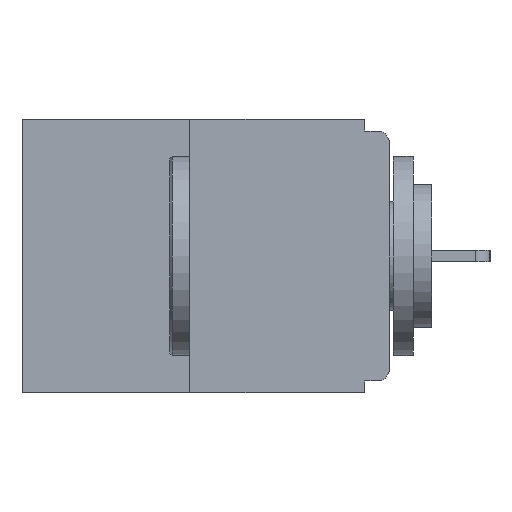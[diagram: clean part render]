
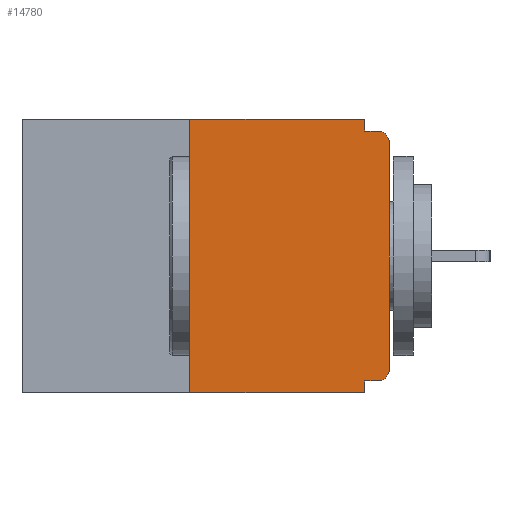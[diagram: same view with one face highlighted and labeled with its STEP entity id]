
A CAD part, left-side view. The second image highlights one B-rep face of the part: STEP entity #14780.
In plain terms, the highlighted planar face has unit normal (-1, 0, 0).
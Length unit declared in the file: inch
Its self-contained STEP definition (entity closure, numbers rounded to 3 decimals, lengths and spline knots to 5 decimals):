
#3 = EDGE_CURVE ( 'NONE', #1493, #1926, #19079, .T. ) ;
#539 = LINE ( 'NONE', #24340, #20192 ) ;
#793 = VECTOR ( 'NONE', #6854, 39.37008 ) ;
#969 = DIRECTION ( 'NONE',  ( 0., 0., 1. ) ) ;
#1248 = DIRECTION ( 'NONE',  ( 0., -1., 0. ) ) ;
#1493 = VERTEX_POINT ( 'NONE', #18992 ) ;
#1844 = EDGE_LOOP ( 'NONE', ( #14877, #3896, #26141, #13266, #27011, #18038, #16383, #17602, #20513, #16211 ) ) ;
#1926 = VERTEX_POINT ( 'NONE', #19876 ) ;
#2379 = CARTESIAN_POINT ( 'NONE',  ( 0., 0., 0. ) ) ;
#3303 = EDGE_CURVE ( 'NONE', #9824, #17893, #20663, .T. ) ;
#3896 = ORIENTED_EDGE ( 'NONE', *, *, #7322, .F. ) ;
#4046 = VECTOR ( 'NONE', #969, 39.37008 ) ;
#4457 = LINE ( 'NONE', #2379, #17481 ) ;
#4623 = LINE ( 'NONE', #19456, #793 ) ;
#4707 = EDGE_CURVE ( 'NONE', #23643, #7368, #18826, .T. ) ;
#4752 = CARTESIAN_POINT ( 'NONE',  ( 0., 0.46, -0.343 ) ) ;
#5246 = CARTESIAN_POINT ( 'NONE',  ( 0., 0.031, -0.343 ) ) ;
#6122 = CARTESIAN_POINT ( 'NONE',  ( 0., 0.25, -0.343 ) ) ;
#6854 = DIRECTION ( 'NONE',  ( 0., -1., 0. ) ) ;
#7193 = CARTESIAN_POINT ( 'NONE',  ( 0., 0.25, 0. ) ) ;
#7202 = FACE_OUTER_BOUND ( 'NONE', #1844, .T. ) ;
#7322 = EDGE_CURVE ( 'NONE', #18952, #11484, #26138, .T. ) ;
#7368 = VERTEX_POINT ( 'NONE', #16182 ) ;
#7459 = DIRECTION ( 'NONE',  ( 0., 0., -1. ) ) ;
#7588 = DIRECTION ( 'NONE',  ( 0., 0., -1. ) ) ;
#7780 = DIRECTION ( 'NONE',  ( 0., 0., -1. ) ) ;
#8576 = VECTOR ( 'NONE', #11274, 39.37008 ) ;
#9267 = EDGE_CURVE ( 'NONE', #18952, #16639, #23722, .T. ) ;
#9301 = PLANE ( 'NONE',  #16674 ) ;
#9710 = DIRECTION ( 'NONE',  ( 1., 0., 0. ) ) ;
#9824 = VERTEX_POINT ( 'NONE', #13534 ) ;
#10579 = AXIS2_PLACEMENT_3D ( 'NONE', #13012, #18964, #21420 ) ;
#10654 = VECTOR ( 'NONE', #14390, 39.37008 ) ;
#11274 = DIRECTION ( 'NONE',  ( 0., -1., 0. ) ) ;
#11484 = VERTEX_POINT ( 'NONE', #15438 ) ;
#11905 = CARTESIAN_POINT ( 'NONE',  ( 0., 0.015, -0.03 ) ) ;
#11906 = CIRCLE ( 'NONE', #10579, 0.015 ) ;
#12388 = CARTESIAN_POINT ( 'NONE',  ( 0., 0.031, 0. ) ) ;
#13012 = CARTESIAN_POINT ( 'NONE',  ( 0., 0.015, -0.313 ) ) ;
#13266 = ORIENTED_EDGE ( 'NONE', *, *, #25120, .F. ) ;
#13534 = CARTESIAN_POINT ( 'NONE',  ( 0., 0.031, 0. ) ) ;
#13606 = VECTOR ( 'NONE', #7780, 39.37008 ) ;
#14097 = DIRECTION ( 'NONE',  ( -1., 0., 0. ) ) ;
#14187 = EDGE_CURVE ( 'NONE', #17893, #1926, #22284, .T. ) ;
#14390 = DIRECTION ( 'NONE',  ( 0., 1., 0. ) ) ;
#14780 = ADVANCED_FACE ( 'NONE', ( #7202 ), #9301, .F. ) ;
#14877 = ORIENTED_EDGE ( 'NONE', *, *, #20833, .F. ) ;
#15438 = CARTESIAN_POINT ( 'NONE',  ( 0., 0.25, 0. ) ) ;
#15499 = CARTESIAN_POINT ( 'NONE',  ( 0., 0.46, 0. ) ) ;
#15529 = AXIS2_PLACEMENT_3D ( 'NONE', #11905, #14097, #7459 ) ;
#15536 = CARTESIAN_POINT ( 'NONE',  ( 0., 0.031, -0.015 ) ) ;
#16182 = CARTESIAN_POINT ( 'NONE',  ( 0., 0.031, -0.328 ) ) ;
#16205 = CARTESIAN_POINT ( 'NONE',  ( 0., 0., -0.328 ) ) ;
#16211 = ORIENTED_EDGE ( 'NONE', *, *, #3303, .F. ) ;
#16383 = ORIENTED_EDGE ( 'NONE', *, *, #18303, .T. ) ;
#16639 = VERTEX_POINT ( 'NONE', #5246 ) ;
#16674 = AXIS2_PLACEMENT_3D ( 'NONE', #15499, #9710, #24375 ) ;
#17481 = VECTOR ( 'NONE', #19681, 39.37008 ) ;
#17602 = ORIENTED_EDGE ( 'NONE', *, *, #3, .T. ) ;
#17893 = VERTEX_POINT ( 'NONE', #15536 ) ;
#18038 = ORIENTED_EDGE ( 'NONE', *, *, #23306, .T. ) ;
#18303 = EDGE_CURVE ( 'NONE', #21466, #1493, #4457, .T. ) ;
#18826 = LINE ( 'NONE', #16205, #10654 ) ;
#18952 = VERTEX_POINT ( 'NONE', #6122 ) ;
#18964 = DIRECTION ( 'NONE',  ( -1., 0., 0. ) ) ;
#18992 = CARTESIAN_POINT ( 'NONE',  ( 0., 0., -0.03 ) ) ;
#19079 = CIRCLE ( 'NONE', #15529, 0.015 ) ;
#19456 = CARTESIAN_POINT ( 'NONE',  ( 0., 0.46, 0. ) ) ;
#19681 = DIRECTION ( 'NONE',  ( 0., 0., 1. ) ) ;
#19876 = CARTESIAN_POINT ( 'NONE',  ( 0., 0.015, -0.015 ) ) ;
#20192 = VECTOR ( 'NONE', #7588, 39.37008 ) ;
#20208 = CARTESIAN_POINT ( 'NONE',  ( 0., 0., -0.015 ) ) ;
#20513 = ORIENTED_EDGE ( 'NONE', *, *, #14187, .F. ) ;
#20663 = LINE ( 'NONE', #12388, #13606 ) ;
#20833 = EDGE_CURVE ( 'NONE', #11484, #9824, #4623, .T. ) ;
#21420 = DIRECTION ( 'NONE',  ( 0., 0., -1. ) ) ;
#21466 = VERTEX_POINT ( 'NONE', #25469 ) ;
#22284 = LINE ( 'NONE', #20208, #25904 ) ;
#23306 = EDGE_CURVE ( 'NONE', #23643, #21466, #11906, .T. ) ;
#23643 = VERTEX_POINT ( 'NONE', #25817 ) ;
#23722 = LINE ( 'NONE', #4752, #8576 ) ;
#24340 = CARTESIAN_POINT ( 'NONE',  ( 0., 0.031, -0.343 ) ) ;
#24375 = DIRECTION ( 'NONE',  ( 0., 0., -1. ) ) ;
#25120 = EDGE_CURVE ( 'NONE', #7368, #16639, #539, .T. ) ;
#25469 = CARTESIAN_POINT ( 'NONE',  ( 0., 0., -0.313 ) ) ;
#25817 = CARTESIAN_POINT ( 'NONE',  ( 0., 0.015, -0.328 ) ) ;
#25904 = VECTOR ( 'NONE', #1248, 39.37008 ) ;
#26138 = LINE ( 'NONE', #7193, #4046 ) ;
#26141 = ORIENTED_EDGE ( 'NONE', *, *, #9267, .T. ) ;
#27011 = ORIENTED_EDGE ( 'NONE', *, *, #4707, .F. ) ;
